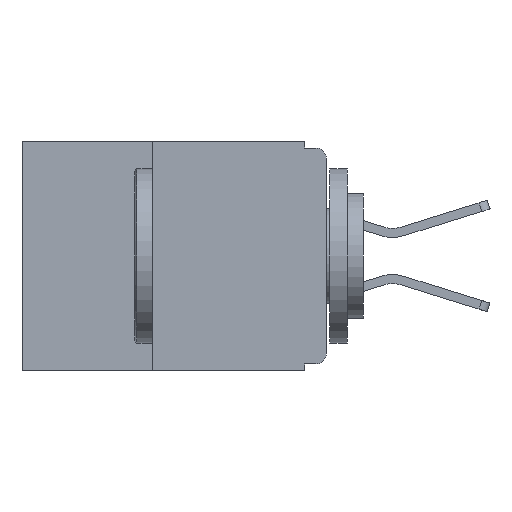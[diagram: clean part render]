
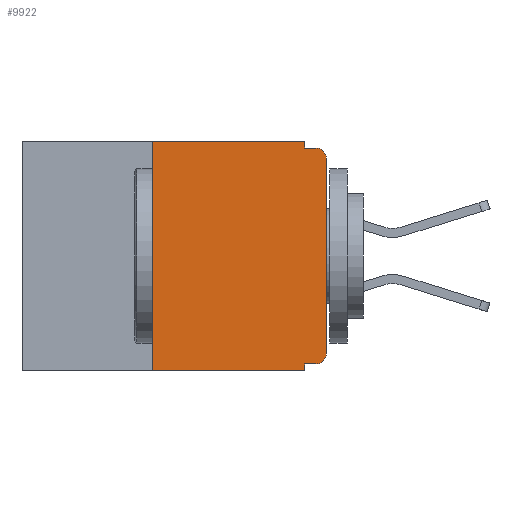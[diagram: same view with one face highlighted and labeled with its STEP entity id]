
A CAD part, left-side view. The second image highlights one B-rep face of the part: STEP entity #9922.
In plain terms, the highlighted planar face has unit normal (-1, 0, 0).
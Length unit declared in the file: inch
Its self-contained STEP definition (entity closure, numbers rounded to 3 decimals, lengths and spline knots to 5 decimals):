
#181 = EDGE_CURVE ( 'NONE', #13957, #2249, #19494, .T. ) ;
#270 = VERTEX_POINT ( 'NONE', #15114 ) ;
#379 = LINE ( 'NONE', #20378, #9333 ) ;
#465 = ORIENTED_EDGE ( 'NONE', *, *, #20808, .F. ) ;
#829 = DIRECTION ( 'NONE',  ( 0., 0., 1. ) ) ;
#883 = CARTESIAN_POINT ( 'NONE',  ( 0., 0.437, 0. ) ) ;
#984 = DIRECTION ( 'NONE',  ( 0., 1., 0. ) ) ;
#988 = CARTESIAN_POINT ( 'NONE',  ( 0., 0., -0.305 ) ) ;
#1064 = CARTESIAN_POINT ( 'NONE',  ( 0., 0., 0. ) ) ;
#1383 = LINE ( 'NONE', #11569, #20012 ) ;
#1395 = DIRECTION ( 'NONE',  ( 0., 0., 1. ) ) ;
#1631 = VECTOR ( 'NONE', #1395, 39.37008 ) ;
#1687 = EDGE_CURVE ( 'NONE', #13560, #13957, #379, .T. ) ;
#2249 = VERTEX_POINT ( 'NONE', #18174 ) ;
#2636 = ORIENTED_EDGE ( 'NONE', *, *, #23178, .F. ) ;
#2728 = DIRECTION ( 'NONE',  ( 0., 0., -1. ) ) ;
#2868 = VECTOR ( 'NONE', #984, 39.37008 ) ;
#3154 = VERTEX_POINT ( 'NONE', #988 ) ;
#3881 = DIRECTION ( 'NONE',  ( -1., 0., 0. ) ) ;
#4620 = CARTESIAN_POINT ( 'NONE',  ( 0., 0.25, -0.33 ) ) ;
#4679 = FACE_OUTER_BOUND ( 'NONE', #11525, .T. ) ;
#5011 = VECTOR ( 'NONE', #13788, 39.37008 ) ;
#5351 = EDGE_CURVE ( 'NONE', #3154, #22966, #6259, .T. ) ;
#5388 = ORIENTED_EDGE ( 'NONE', *, *, #1687, .F. ) ;
#5394 = CIRCLE ( 'NONE', #5924, 0.015 ) ;
#5673 = CARTESIAN_POINT ( 'NONE',  ( 0., 0.031, -0.01 ) ) ;
#5924 = AXIS2_PLACEMENT_3D ( 'NONE', #15030, #3881, #16835 ) ;
#6259 = LINE ( 'NONE', #1064, #20954 ) ;
#6650 = CARTESIAN_POINT ( 'NONE',  ( 0., 0.031, -0.33 ) ) ;
#6720 = DIRECTION ( 'NONE',  ( 1., 0., 0. ) ) ;
#7382 = VERTEX_POINT ( 'NONE', #23416 ) ;
#7562 = CARTESIAN_POINT ( 'NONE',  ( 0., 0.031, 0. ) ) ;
#7733 = CARTESIAN_POINT ( 'NONE',  ( 0., 0.25, 0. ) ) ;
#9293 = AXIS2_PLACEMENT_3D ( 'NONE', #9873, #22639, #11812 ) ;
#9333 = VECTOR ( 'NONE', #2728, 39.37008 ) ;
#9717 = VECTOR ( 'NONE', #18387, 39.37008 ) ;
#9873 = CARTESIAN_POINT ( 'NONE',  ( 0., 0.015, -0.025 ) ) ;
#9922 = ADVANCED_FACE ( 'NONE', ( #4679 ), #17800, .F. ) ;
#10613 = ORIENTED_EDGE ( 'NONE', *, *, #19465, .F. ) ;
#10829 = CARTESIAN_POINT ( 'NONE',  ( 0., 0.25, -0.33 ) ) ;
#11307 = ORIENTED_EDGE ( 'NONE', *, *, #17014, .T. ) ;
#11525 = EDGE_LOOP ( 'NONE', ( #15581, #11307, #16723, #5388, #21244, #2636, #18055, #465, #10613, #20884 ) ) ;
#11569 = CARTESIAN_POINT ( 'NONE',  ( 0., 0.437, -0.33 ) ) ;
#11812 = DIRECTION ( 'NONE',  ( 0., 0., -1. ) ) ;
#12891 = LINE ( 'NONE', #14193, #2868 ) ;
#13560 = VERTEX_POINT ( 'NONE', #7562 ) ;
#13788 = DIRECTION ( 'NONE',  ( 0., 0., -1. ) ) ;
#13957 = VERTEX_POINT ( 'NONE', #5673 ) ;
#14186 = AXIS2_PLACEMENT_3D ( 'NONE', #883, #6720, #19646 ) ;
#14193 = CARTESIAN_POINT ( 'NONE',  ( 0., 0., -0.32 ) ) ;
#14612 = EDGE_CURVE ( 'NONE', #7382, #3154, #5394, .T. ) ;
#15030 = CARTESIAN_POINT ( 'NONE',  ( 0., 0.015, -0.305 ) ) ;
#15114 = CARTESIAN_POINT ( 'NONE',  ( 0., 0.031, -0.32 ) ) ;
#15581 = ORIENTED_EDGE ( 'NONE', *, *, #5351, .T. ) ;
#16083 = CARTESIAN_POINT ( 'NONE',  ( 0., 0.437, 0. ) ) ;
#16551 = LINE ( 'NONE', #10829, #1631 ) ;
#16723 = ORIENTED_EDGE ( 'NONE', *, *, #181, .F. ) ;
#16835 = DIRECTION ( 'NONE',  ( 0., 0., -1. ) ) ;
#17014 = EDGE_CURVE ( 'NONE', #22966, #2249, #20362, .T. ) ;
#17047 = DIRECTION ( 'NONE',  ( 0., -1., 0. ) ) ;
#17269 = VERTEX_POINT ( 'NONE', #6650 ) ;
#17324 = EDGE_CURVE ( 'NONE', #22697, #13560, #19495, .T. ) ;
#17399 = CARTESIAN_POINT ( 'NONE',  ( 0., 0.031, -0.33 ) ) ;
#17800 = PLANE ( 'NONE',  #14186 ) ;
#17901 = DIRECTION ( 'NONE',  ( 0., -1., 0. ) ) ;
#18055 = ORIENTED_EDGE ( 'NONE', *, *, #22006, .T. ) ;
#18174 = CARTESIAN_POINT ( 'NONE',  ( 0., 0.015, -0.01 ) ) ;
#18387 = DIRECTION ( 'NONE',  ( 0., -1., 0. ) ) ;
#18964 = VECTOR ( 'NONE', #17901, 39.37008 ) ;
#19374 = VERTEX_POINT ( 'NONE', #4620 ) ;
#19465 = EDGE_CURVE ( 'NONE', #7382, #270, #12891, .T. ) ;
#19494 = LINE ( 'NONE', #20038, #9717 ) ;
#19495 = LINE ( 'NONE', #16083, #18964 ) ;
#19646 = DIRECTION ( 'NONE',  ( 0., 0., -1. ) ) ;
#19772 = LINE ( 'NONE', #17399, #5011 ) ;
#20012 = VECTOR ( 'NONE', #17047, 39.37008 ) ;
#20038 = CARTESIAN_POINT ( 'NONE',  ( 0., 0., -0.01 ) ) ;
#20362 = CIRCLE ( 'NONE', #9293, 0.015 ) ;
#20378 = CARTESIAN_POINT ( 'NONE',  ( 0., 0.031, 0. ) ) ;
#20808 = EDGE_CURVE ( 'NONE', #270, #17269, #19772, .T. ) ;
#20884 = ORIENTED_EDGE ( 'NONE', *, *, #14612, .T. ) ;
#20954 = VECTOR ( 'NONE', #829, 39.37008 ) ;
#21244 = ORIENTED_EDGE ( 'NONE', *, *, #17324, .F. ) ;
#22006 = EDGE_CURVE ( 'NONE', #19374, #17269, #1383, .T. ) ;
#22639 = DIRECTION ( 'NONE',  ( -1., 0., 0. ) ) ;
#22697 = VERTEX_POINT ( 'NONE', #7733 ) ;
#22901 = CARTESIAN_POINT ( 'NONE',  ( 0., 0., -0.025 ) ) ;
#22966 = VERTEX_POINT ( 'NONE', #22901 ) ;
#23178 = EDGE_CURVE ( 'NONE', #19374, #22697, #16551, .T. ) ;
#23416 = CARTESIAN_POINT ( 'NONE',  ( 0., 0.015, -0.32 ) ) ;
